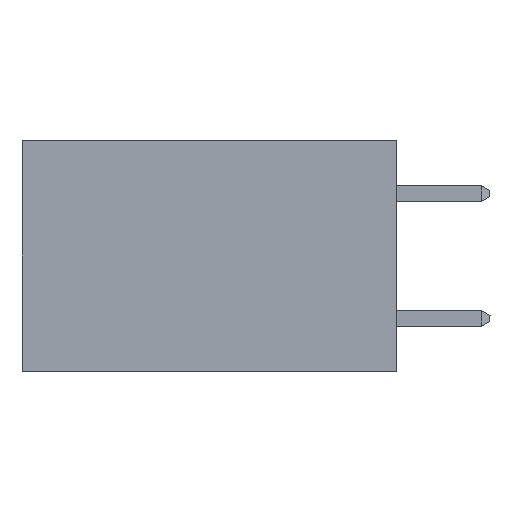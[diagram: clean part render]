
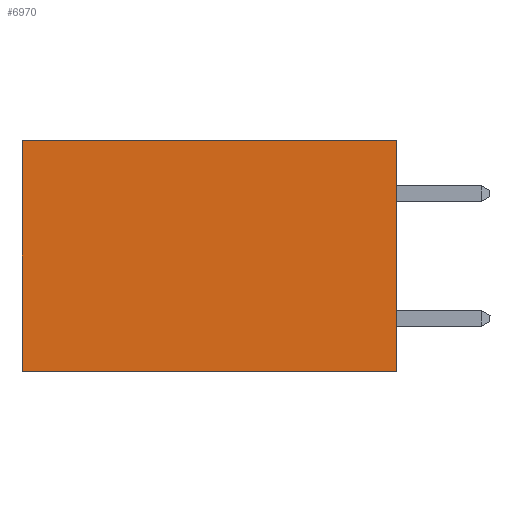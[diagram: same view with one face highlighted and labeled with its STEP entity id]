
A CAD part, left-side view. The second image highlights one B-rep face of the part: STEP entity #6970.
In plain terms, the highlighted planar face has unit normal (-1, 0, 0).
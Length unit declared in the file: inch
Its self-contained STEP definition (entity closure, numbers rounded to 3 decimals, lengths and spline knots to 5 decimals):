
#761 = VERTEX_POINT ( 'NONE', #11303 ) ;
#810 = LINE ( 'NONE', #7051, #7138 ) ;
#1964 = CARTESIAN_POINT ( 'NONE',  ( 0.298, 0.6, 0. ) ) ;
#2159 = VERTEX_POINT ( 'NONE', #3114 ) ;
#2429 = ORIENTED_EDGE ( 'NONE', *, *, #11434, .T. ) ;
#2989 = ORIENTED_EDGE ( 'NONE', *, *, #3741, .T. ) ;
#3104 = ORIENTED_EDGE ( 'NONE', *, *, #11509, .F. ) ;
#3105 = ORIENTED_EDGE ( 'NONE', *, *, #7155, .F. ) ;
#3114 = CARTESIAN_POINT ( 'NONE',  ( 0.298, 0.6, 0. ) ) ;
#3144 = LINE ( 'NONE', #10558, #7783 ) ;
#3741 = EDGE_CURVE ( 'NONE', #2159, #761, #9772, .T. ) ;
#4358 = VERTEX_POINT ( 'NONE', #9764 ) ;
#4696 = AXIS2_PLACEMENT_3D ( 'NONE', #9690, #9734, #5200 ) ;
#5077 = DIRECTION ( 'NONE',  ( 0., 1., 0. ) ) ;
#5200 = DIRECTION ( 'NONE',  ( 0., 0., -1. ) ) ;
#6369 = VECTOR ( 'NONE', #10515, 39.37008 ) ;
#6791 = VECTOR ( 'NONE', #8206, 39.37008 ) ;
#6970 = ADVANCED_FACE ( 'NONE', ( #10519 ), #9650, .F. ) ;
#7051 = CARTESIAN_POINT ( 'NONE',  ( 0.298, 0., 0. ) ) ;
#7061 = VERTEX_POINT ( 'NONE', #11572 ) ;
#7138 = VECTOR ( 'NONE', #7400, 39.37008 ) ;
#7155 = EDGE_CURVE ( 'NONE', #4358, #7061, #810, .T. ) ;
#7400 = DIRECTION ( 'NONE',  ( 0., 0., -1. ) ) ;
#7783 = VECTOR ( 'NONE', #5077, 39.37008 ) ;
#8206 = DIRECTION ( 'NONE',  ( 0., 0., -1. ) ) ;
#8624 = CARTESIAN_POINT ( 'NONE',  ( 0.298, 0., -0.37 ) ) ;
#8830 = EDGE_LOOP ( 'NONE', ( #2989, #3104, #3105, #2429 ) ) ;
#9650 = PLANE ( 'NONE',  #4696 ) ;
#9690 = CARTESIAN_POINT ( 'NONE',  ( 0.298, 0., 0. ) ) ;
#9734 = DIRECTION ( 'NONE',  ( 1., 0., 0. ) ) ;
#9764 = CARTESIAN_POINT ( 'NONE',  ( 0.298, 0., 0. ) ) ;
#9772 = LINE ( 'NONE', #1964, #6791 ) ;
#10169 = LINE ( 'NONE', #8624, #6369 ) ;
#10515 = DIRECTION ( 'NONE',  ( 0., 1., 0. ) ) ;
#10519 = FACE_OUTER_BOUND ( 'NONE', #8830, .T. ) ;
#10558 = CARTESIAN_POINT ( 'NONE',  ( 0.298, 0., 0. ) ) ;
#11303 = CARTESIAN_POINT ( 'NONE',  ( 0.298, 0.6, -0.37 ) ) ;
#11434 = EDGE_CURVE ( 'NONE', #4358, #2159, #3144, .T. ) ;
#11509 = EDGE_CURVE ( 'NONE', #7061, #761, #10169, .T. ) ;
#11572 = CARTESIAN_POINT ( 'NONE',  ( 0.298, 0., -0.37 ) ) ;
